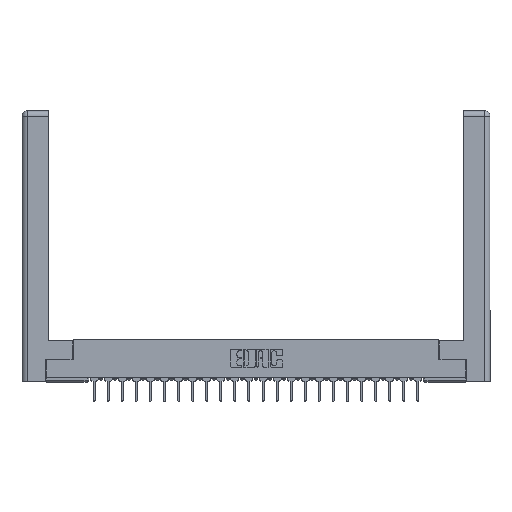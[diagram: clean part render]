
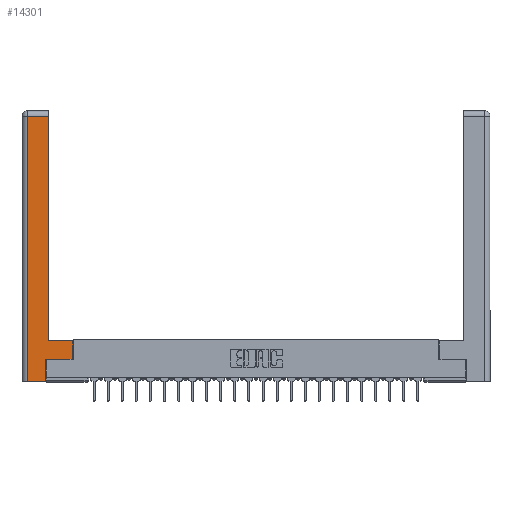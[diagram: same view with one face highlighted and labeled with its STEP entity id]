
A CAD part, top view. The second image highlights one B-rep face of the part: STEP entity #14301.
In plain terms, the highlighted planar face has unit normal (0, 0, 1).
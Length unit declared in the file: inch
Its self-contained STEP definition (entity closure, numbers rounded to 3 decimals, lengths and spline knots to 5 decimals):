
#213 = VERTEX_POINT ( 'NONE', #2446 ) ;
#222 = CARTESIAN_POINT ( 'NONE',  ( 0.565, 0.245, 0. ) ) ;
#706 = LINE ( 'NONE', #21237, #20297 ) ;
#876 = CARTESIAN_POINT ( 'NONE',  ( 0.295, 0.45, 0. ) ) ;
#1230 = ORIENTED_EDGE ( 'NONE', *, *, #5286, .T. ) ;
#1367 = CARTESIAN_POINT ( 'NONE',  ( 0.265, 0.245, 0. ) ) ;
#1634 = CARTESIAN_POINT ( 'NONE',  ( 0.265, 0., 0. ) ) ;
#1657 = CARTESIAN_POINT ( 'NONE',  ( 0.565, 0.45, 0. ) ) ;
#2054 = VERTEX_POINT ( 'NONE', #23774 ) ;
#2446 = CARTESIAN_POINT ( 'NONE',  ( 0.295, 2.94, 0. ) ) ;
#2622 = DIRECTION ( 'NONE',  ( -1., 0., 0. ) ) ;
#2734 = ORIENTED_EDGE ( 'NONE', *, *, #25142, .T. ) ;
#2809 = CARTESIAN_POINT ( 'NONE',  ( 0., 0., 0. ) ) ;
#3105 = DIRECTION ( 'NONE',  ( -1., 0., 0. ) ) ;
#3245 = DIRECTION ( 'NONE',  ( 1., 0., 0. ) ) ;
#3511 = DIRECTION ( 'NONE',  ( 1., 0., 0. ) ) ;
#3538 = EDGE_CURVE ( 'NONE', #15656, #17099, #20042, .T. ) ;
#3646 = CARTESIAN_POINT ( 'NONE',  ( 0.565, 0.45, 0. ) ) ;
#3950 = CARTESIAN_POINT ( 'NONE',  ( 0.0615, 0., 0. ) ) ;
#4875 = CARTESIAN_POINT ( 'NONE',  ( 0.0615, 2.94, 0. ) ) ;
#5286 = EDGE_CURVE ( 'NONE', #2054, #213, #21128, .T. ) ;
#5877 = ORIENTED_EDGE ( 'NONE', *, *, #19814, .T. ) ;
#6537 = DIRECTION ( 'NONE',  ( -1., 0., 0. ) ) ;
#6598 = VERTEX_POINT ( 'NONE', #222 ) ;
#6707 = VERTEX_POINT ( 'NONE', #4875 ) ;
#6825 = CARTESIAN_POINT ( 'NONE',  ( 0.265, 0., 0. ) ) ;
#7227 = CARTESIAN_POINT ( 'NONE',  ( 0.565, 0.245, 0. ) ) ;
#7754 = VECTOR ( 'NONE', #13805, 39.37008 ) ;
#8556 = VECTOR ( 'NONE', #3245, 39.37008 ) ;
#9985 = EDGE_CURVE ( 'NONE', #17099, #6598, #11851, .T. ) ;
#11055 = ORIENTED_EDGE ( 'NONE', *, *, #9985, .T. ) ;
#11082 = CARTESIAN_POINT ( 'NONE',  ( 0.295, 3., 0. ) ) ;
#11134 = VECTOR ( 'NONE', #3511, 39.37008 ) ;
#11816 = ORIENTED_EDGE ( 'NONE', *, *, #16694, .T. ) ;
#11824 = VECTOR ( 'NONE', #21917, 39.37008 ) ;
#11851 = LINE ( 'NONE', #7227, #8556 ) ;
#12371 = ORIENTED_EDGE ( 'NONE', *, *, #12677, .T. ) ;
#12677 = EDGE_CURVE ( 'NONE', #19703, #2054, #12792, .T. ) ;
#12792 = LINE ( 'NONE', #876, #15212 ) ;
#12813 = LINE ( 'NONE', #15058, #15456 ) ;
#13805 = DIRECTION ( 'NONE',  ( 0., 1., 0. ) ) ;
#14301 = ADVANCED_FACE ( 'NONE', ( #20947 ), #16573, .F. ) ;
#15058 = CARTESIAN_POINT ( 'NONE',  ( 0.0615, 0., 0. ) ) ;
#15150 = AXIS2_PLACEMENT_3D ( 'NONE', #2809, #18546, #6537 ) ;
#15212 = VECTOR ( 'NONE', #2622, 39.37008 ) ;
#15456 = VECTOR ( 'NONE', #25007, 39.37008 ) ;
#15656 = VERTEX_POINT ( 'NONE', #6825 ) ;
#15715 = EDGE_CURVE ( 'NONE', #213, #6707, #706, .T. ) ;
#16573 = PLANE ( 'NONE',  #15150 ) ;
#16694 = EDGE_CURVE ( 'NONE', #6598, #19703, #25902, .T. ) ;
#17099 = VERTEX_POINT ( 'NONE', #1367 ) ;
#17637 = DIRECTION ( 'NONE',  ( 0., 1., 0. ) ) ;
#18452 = CARTESIAN_POINT ( 'NONE',  ( 0.265, 0.245, 0. ) ) ;
#18546 = DIRECTION ( 'NONE',  ( 0., 0., -1. ) ) ;
#19703 = VERTEX_POINT ( 'NONE', #3646 ) ;
#19814 = EDGE_CURVE ( 'NONE', #20567, #15656, #23906, .T. ) ;
#20042 = LINE ( 'NONE', #18452, #7754 ) ;
#20297 = VECTOR ( 'NONE', #3105, 39.37008 ) ;
#20567 = VERTEX_POINT ( 'NONE', #3950 ) ;
#20947 = FACE_OUTER_BOUND ( 'NONE', #24836, .T. ) ;
#21128 = LINE ( 'NONE', #11082, #23853 ) ;
#21237 = CARTESIAN_POINT ( 'NONE',  ( 0.0615, 2.94, 0. ) ) ;
#21917 = DIRECTION ( 'NONE',  ( 0., 1., 0. ) ) ;
#22334 = ORIENTED_EDGE ( 'NONE', *, *, #15715, .T. ) ;
#23009 = ORIENTED_EDGE ( 'NONE', *, *, #3538, .T. ) ;
#23774 = CARTESIAN_POINT ( 'NONE',  ( 0.295, 0.45, 0. ) ) ;
#23853 = VECTOR ( 'NONE', #17637, 39.37008 ) ;
#23906 = LINE ( 'NONE', #1634, #11134 ) ;
#24836 = EDGE_LOOP ( 'NONE', ( #1230, #22334, #2734, #5877, #23009, #11055, #11816, #12371 ) ) ;
#25007 = DIRECTION ( 'NONE',  ( 0., -1., 0. ) ) ;
#25142 = EDGE_CURVE ( 'NONE', #6707, #20567, #12813, .T. ) ;
#25902 = LINE ( 'NONE', #1657, #11824 ) ;
